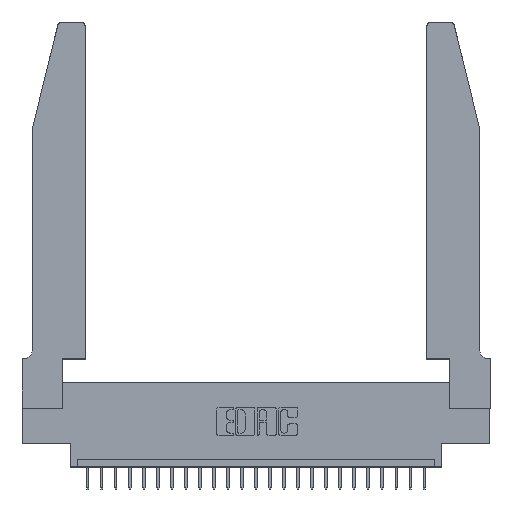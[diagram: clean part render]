
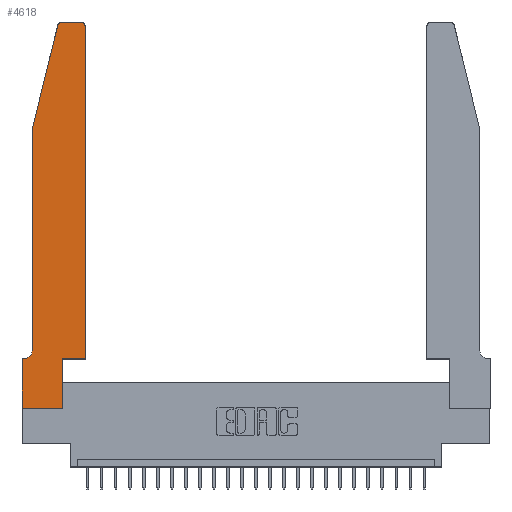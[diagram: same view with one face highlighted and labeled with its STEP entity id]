
A CAD part, top view. The second image highlights one B-rep face of the part: STEP entity #4618.
In plain terms, the highlighted planar face has unit normal (0, 0, 1).
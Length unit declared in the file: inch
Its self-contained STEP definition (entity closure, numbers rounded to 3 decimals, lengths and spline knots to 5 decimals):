
#229 = CARTESIAN_POINT ( 'NONE',  ( 0.0755, 2., 0.37 ) ) ;
#308 = CARTESIAN_POINT ( 'NONE',  ( 0.4205, 2.75, 0.37 ) ) ;
#588 = ORIENTED_EDGE ( 'NONE', *, *, #22257, .T. ) ;
#625 = VERTEX_POINT ( 'NONE', #229 ) ;
#702 = DIRECTION ( 'NONE',  ( 1., 0., 0. ) ) ;
#792 = CARTESIAN_POINT ( 'NONE',  ( 0., 0., 0.37 ) ) ;
#1193 = ORIENTED_EDGE ( 'NONE', *, *, #19273, .T. ) ;
#1320 = VECTOR ( 'NONE', #4790, 39.37008 ) ;
#2327 = DIRECTION ( 'NONE',  ( 1., 0., 0. ) ) ;
#2889 = VERTEX_POINT ( 'NONE', #14364 ) ;
#3010 = ORIENTED_EDGE ( 'NONE', *, *, #8995, .T. ) ;
#3031 = CIRCLE ( 'NONE', #9488, 0.03 ) ;
#3494 = CARTESIAN_POINT ( 'NONE',  ( 0.0755, 2., 0.37 ) ) ;
#3850 = DIRECTION ( 'NONE',  ( -0.239, -0.971, 0. ) ) ;
#4618 = ADVANCED_FACE ( 'NONE', ( #20835 ), #20708, .T. ) ;
#4790 = DIRECTION ( 'NONE',  ( 0., -1., 0. ) ) ;
#5040 = CARTESIAN_POINT ( 'NONE',  ( 0.0755, 2., 0.37 ) ) ;
#5060 = VERTEX_POINT ( 'NONE', #19804 ) ;
#5079 = VERTEX_POINT ( 'NONE', #8924 ) ;
#5371 = VECTOR ( 'NONE', #3850, 39.37008 ) ;
#5546 = ORIENTED_EDGE ( 'NONE', *, *, #10008, .T. ) ;
#5592 = AXIS2_PLACEMENT_3D ( 'NONE', #8344, #8598, #2327 ) ;
#5872 = VECTOR ( 'NONE', #7720, 39.37008 ) ;
#6158 = VERTEX_POINT ( 'NONE', #23131 ) ;
#6207 = DIRECTION ( 'NONE',  ( 0., 1., 0. ) ) ;
#6543 = CIRCLE ( 'NONE', #5592, 0.03 ) ;
#7009 = LINE ( 'NONE', #5040, #1320 ) ;
#7720 = DIRECTION ( 'NONE',  ( 0., -1., 0. ) ) ;
#8304 = LINE ( 'NONE', #17806, #17723 ) ;
#8344 = CARTESIAN_POINT ( 'NONE',  ( 0.284, 2.72, 0.37 ) ) ;
#8598 = DIRECTION ( 'NONE',  ( 0., 0., 1. ) ) ;
#8683 = ORIENTED_EDGE ( 'NONE', *, *, #17759, .T. ) ;
#8924 = CARTESIAN_POINT ( 'NONE',  ( 0.284, 2.75, 0.37 ) ) ;
#8995 = EDGE_CURVE ( 'NONE', #625, #5060, #7009, .T. ) ;
#9017 = VERTEX_POINT ( 'NONE', #13521 ) ;
#9488 = AXIS2_PLACEMENT_3D ( 'NONE', #23826, #17761, #25842 ) ;
#9777 = DIRECTION ( 'NONE',  ( 1., 0., 0. ) ) ;
#9984 = CARTESIAN_POINT ( 'NONE',  ( 0.0055, 0.42, 0.37 ) ) ;
#10008 = EDGE_CURVE ( 'NONE', #17358, #625, #15416, .T. ) ;
#10084 = CARTESIAN_POINT ( 'NONE',  ( 0., 0., 0.37 ) ) ;
#10133 = ORIENTED_EDGE ( 'NONE', *, *, #15530, .T. ) ;
#11084 = CARTESIAN_POINT ( 'NONE',  ( 0.0055, 0.35, 0.37 ) ) ;
#11902 = LINE ( 'NONE', #14522, #16955 ) ;
#12230 = CARTESIAN_POINT ( 'NONE',  ( 0.2865, 0.35, 0.37 ) ) ;
#12679 = CARTESIAN_POINT ( 'NONE',  ( 0.4505, 0.35, 0.37 ) ) ;
#12857 = VERTEX_POINT ( 'NONE', #10084 ) ;
#12965 = DIRECTION ( 'NONE',  ( 0., 1., 0. ) ) ;
#13255 = CARTESIAN_POINT ( 'NONE',  ( 0.2605, 2.75, 0.37 ) ) ;
#13521 = CARTESIAN_POINT ( 'NONE',  ( 0.2865, 0.35, 0.37 ) ) ;
#14209 = EDGE_CURVE ( 'NONE', #14476, #24176, #18871, .T. ) ;
#14258 = VECTOR ( 'NONE', #17143, 39.37008 ) ;
#14312 = ORIENTED_EDGE ( 'NONE', *, *, #15560, .T. ) ;
#14364 = CARTESIAN_POINT ( 'NONE',  ( 0.2865, 0., 0.37 ) ) ;
#14476 = VERTEX_POINT ( 'NONE', #12679 ) ;
#14522 = CARTESIAN_POINT ( 'NONE',  ( 0.0755, 0.35, 0.37 ) ) ;
#14623 = DIRECTION ( 'NONE',  ( 1., 0., 0. ) ) ;
#14660 = AXIS2_PLACEMENT_3D ( 'NONE', #18851, #18512, #14623 ) ;
#15191 = VECTOR ( 'NONE', #6207, 39.37008 ) ;
#15416 = LINE ( 'NONE', #3494, #5371 ) ;
#15530 = EDGE_CURVE ( 'NONE', #5060, #24213, #23536, .T. ) ;
#15560 = EDGE_CURVE ( 'NONE', #5079, #17358, #6543, .T. ) ;
#16168 = ORIENTED_EDGE ( 'NONE', *, *, #14209, .T. ) ;
#16216 = DIRECTION ( 'NONE',  ( -1., 0., 0. ) ) ;
#16955 = VECTOR ( 'NONE', #16216, 39.37008 ) ;
#16980 = VECTOR ( 'NONE', #12965, 39.37008 ) ;
#17143 = DIRECTION ( 'NONE',  ( -1., 0., 0. ) ) ;
#17358 = VERTEX_POINT ( 'NONE', #24582 ) ;
#17384 = VERTEX_POINT ( 'NONE', #308 ) ;
#17417 = VECTOR ( 'NONE', #702, 39.37008 ) ;
#17723 = VECTOR ( 'NONE', #9777, 39.37008 ) ;
#17759 = EDGE_CURVE ( 'NONE', #9017, #14476, #8304, .T. ) ;
#17761 = DIRECTION ( 'NONE',  ( 0., 0., 1. ) ) ;
#17806 = CARTESIAN_POINT ( 'NONE',  ( 0.4505, 0.35, 0.37 ) ) ;
#17818 = LINE ( 'NONE', #25972, #5872 ) ;
#17892 = EDGE_CURVE ( 'NONE', #2889, #9017, #23390, .T. ) ;
#18261 = DIRECTION ( 'NONE',  ( 0., 0., -1. ) ) ;
#18512 = DIRECTION ( 'NONE',  ( 0., 0., 1. ) ) ;
#18851 = CARTESIAN_POINT ( 'NONE',  ( 0., 0.35, 0.37 ) ) ;
#18871 = LINE ( 'NONE', #22756, #16980 ) ;
#19273 = EDGE_CURVE ( 'NONE', #12857, #2889, #22771, .T. ) ;
#19380 = EDGE_CURVE ( 'NONE', #17384, #5079, #20902, .T. ) ;
#19804 = CARTESIAN_POINT ( 'NONE',  ( 0.0755, 0.42, 0.37 ) ) ;
#20708 = PLANE ( 'NONE',  #14660 ) ;
#20835 = FACE_OUTER_BOUND ( 'NONE', #23045, .T. ) ;
#20902 = LINE ( 'NONE', #13255, #14258 ) ;
#21215 = CARTESIAN_POINT ( 'NONE',  ( 0.4505, 2.72, 0.37 ) ) ;
#21479 = ORIENTED_EDGE ( 'NONE', *, *, #17892, .T. ) ;
#22257 = EDGE_CURVE ( 'NONE', #24213, #6158, #11902, .T. ) ;
#22364 = ORIENTED_EDGE ( 'NONE', *, *, #23884, .T. ) ;
#22685 = ORIENTED_EDGE ( 'NONE', *, *, #23776, .T. ) ;
#22756 = CARTESIAN_POINT ( 'NONE',  ( 0.4505, 0.35, 0.37 ) ) ;
#22771 = LINE ( 'NONE', #792, #17417 ) ;
#23045 = EDGE_LOOP ( 'NONE', ( #25044, #14312, #5546, #3010, #10133, #588, #22364, #1193, #21479, #8683, #16168, #22685 ) ) ;
#23131 = CARTESIAN_POINT ( 'NONE',  ( 0., 0.35, 0.37 ) ) ;
#23390 = LINE ( 'NONE', #12230, #15191 ) ;
#23536 = CIRCLE ( 'NONE', #25777, 0.07 ) ;
#23776 = EDGE_CURVE ( 'NONE', #24176, #17384, #3031, .T. ) ;
#23826 = CARTESIAN_POINT ( 'NONE',  ( 0.4205, 2.72, 0.37 ) ) ;
#23884 = EDGE_CURVE ( 'NONE', #6158, #12857, #17818, .T. ) ;
#24057 = DIRECTION ( 'NONE',  ( -1., 0., 0. ) ) ;
#24176 = VERTEX_POINT ( 'NONE', #21215 ) ;
#24213 = VERTEX_POINT ( 'NONE', #11084 ) ;
#24582 = CARTESIAN_POINT ( 'NONE',  ( 0.25487, 2.72718, 0.37 ) ) ;
#25044 = ORIENTED_EDGE ( 'NONE', *, *, #19380, .T. ) ;
#25777 = AXIS2_PLACEMENT_3D ( 'NONE', #9984, #18261, #24057 ) ;
#25842 = DIRECTION ( 'NONE',  ( 1., 0., 0. ) ) ;
#25972 = CARTESIAN_POINT ( 'NONE',  ( 0., 0., 0.37 ) ) ;
